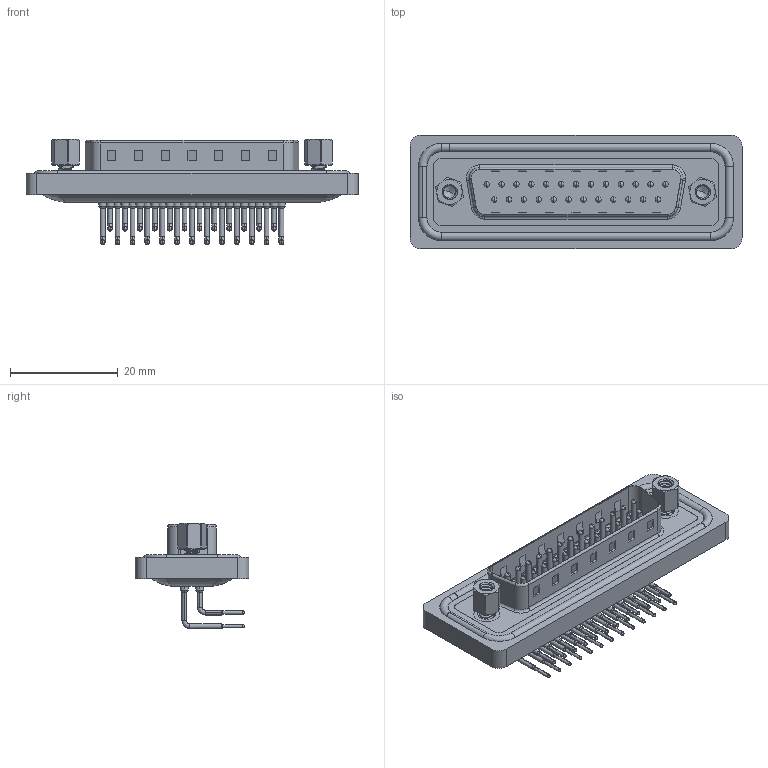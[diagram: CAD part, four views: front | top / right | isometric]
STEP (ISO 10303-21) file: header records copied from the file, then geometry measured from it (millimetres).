
FILE_DESCRIPTION (( 'STEP AP203' ), '1' );
FILE_NAME ('629-W25-240-012.STEP', '2024-04-12T16:15:56', ( '' ), ( '' ), 'SwSTEP 2.0', 'SolidWorks 2023', '' );
FILE_SCHEMA (( 'CONFIG_CONTROL_DESIGN' ));
Length unit declared in the file: millimetre
Products named in the file (8): 629W Housing_25 Contacts; 629W Waterproof Housing_25 Contacts; 629W 4-40 Hex Standoff; 629W 4-40 Threaded Rivet_Stabilizer; 629W Contact Row 2; 629W Shell_25 Contacts; 629W Contact Row 1; 629-W25-240-012
Assembly tree (32 placements, depth 2):
  629-W25-240-012
    629W Housing_25 Contacts
    629W Shell_25 Contacts
    629W Waterproof Housing_25 Contacts
    629W Contact Row 1  x13
    629W Contact Row 2  x12
    629W 4-40 Threaded Rivet_Stabilizer  x2
    629W 4-40 Hex Standoff  x2
Bounding box: 61.74 x 21.1 x 19.59 mm (x, y, z)
Volume: 6426.5 mm3; surface area: 11459.7 mm2
Topology: 33 solids, 33 shells, 3314 faces, 9258 edges, 6021 vertices
Faces by surface type: plane 1805, cylinder 1166, bspline 172, cone 128, torus 43
Entity records: 32703 total; most frequent: CARTESIAN_POINT 9110, DIRECTION 4752, ORIENTED_EDGE 4512, EDGE_CURVE 2256, AXIS2_PLACEMENT_3D 1752, VERTEX_POINT 1467, LINE 1248, VECTOR 1248
